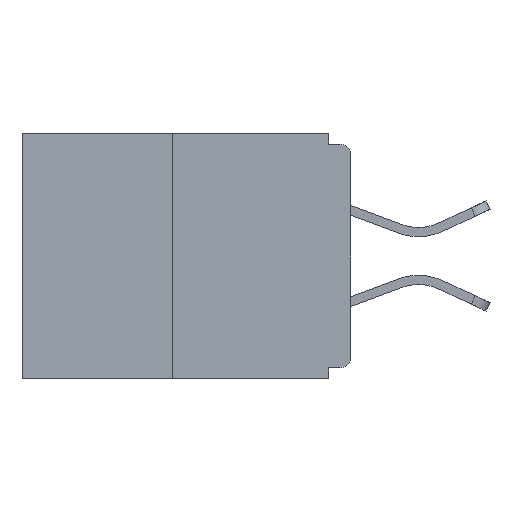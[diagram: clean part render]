
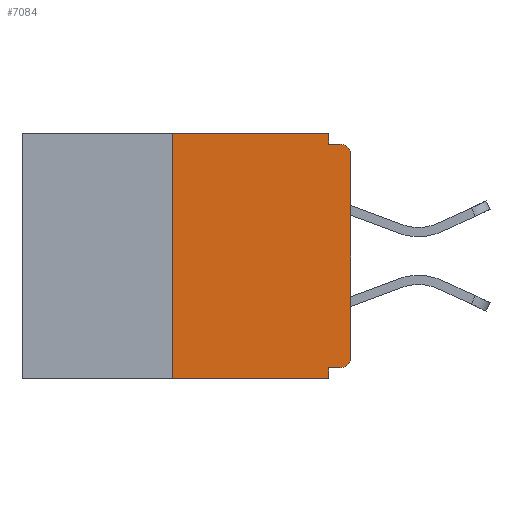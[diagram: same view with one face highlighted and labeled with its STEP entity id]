
A CAD part, left-side view. The second image highlights one B-rep face of the part: STEP entity #7084.
In plain terms, the highlighted planar face has unit normal (-1, 0, 0).
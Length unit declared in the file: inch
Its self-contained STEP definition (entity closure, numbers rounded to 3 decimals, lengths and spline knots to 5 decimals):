
#202 = DIRECTION ( 'NONE',  ( -1., 0., 0. ) ) ;
#292 = ORIENTED_EDGE ( 'NONE', *, *, #16657, .F. ) ;
#450 = EDGE_CURVE ( 'NONE', #7849, #12777, #5446, .T. ) ;
#792 = VECTOR ( 'NONE', #19011, 39.37008 ) ;
#882 = CARTESIAN_POINT ( 'NONE',  ( 0., 0.25, -0.343 ) ) ;
#975 = LINE ( 'NONE', #17782, #13413 ) ;
#1173 = VERTEX_POINT ( 'NONE', #20129 ) ;
#2070 = CARTESIAN_POINT ( 'NONE',  ( 0., 0.25, 0. ) ) ;
#2270 = ORIENTED_EDGE ( 'NONE', *, *, #19446, .T. ) ;
#2441 = LINE ( 'NONE', #14043, #18023 ) ;
#2995 = LINE ( 'NONE', #18815, #792 ) ;
#3107 = CARTESIAN_POINT ( 'NONE',  ( 0., 0.031, -0.015 ) ) ;
#3243 = DIRECTION ( 'NONE',  ( 0., 0., -1. ) ) ;
#3460 = ORIENTED_EDGE ( 'NONE', *, *, #10052, .F. ) ;
#3511 = LINE ( 'NONE', #4772, #19583 ) ;
#3733 = CARTESIAN_POINT ( 'NONE',  ( 0., 0.46, 0. ) ) ;
#3888 = DIRECTION ( 'NONE',  ( 0., -1., 0. ) ) ;
#3919 = VERTEX_POINT ( 'NONE', #2070 ) ;
#4026 = CARTESIAN_POINT ( 'NONE',  ( 0., 0.031, -0.328 ) ) ;
#4136 = CARTESIAN_POINT ( 'NONE',  ( 0., 0.031, -0.343 ) ) ;
#4229 = DIRECTION ( 'NONE',  ( 0., 0., -1. ) ) ;
#4297 = ORIENTED_EDGE ( 'NONE', *, *, #8947, .F. ) ;
#4772 = CARTESIAN_POINT ( 'NONE',  ( 0., 0.25, 0. ) ) ;
#4826 = CARTESIAN_POINT ( 'NONE',  ( 0., 0.015, -0.03 ) ) ;
#5094 = CARTESIAN_POINT ( 'NONE',  ( 0., 0.031, 0. ) ) ;
#5446 = LINE ( 'NONE', #12890, #10282 ) ;
#5510 = DIRECTION ( 'NONE',  ( 0., -1., 0. ) ) ;
#5558 = VERTEX_POINT ( 'NONE', #5094 ) ;
#5846 = DIRECTION ( 'NONE',  ( 0., 0., 1. ) ) ;
#5995 = LINE ( 'NONE', #3733, #7637 ) ;
#7084 = ADVANCED_FACE ( 'NONE', ( #8911 ), #7354, .F. ) ;
#7354 = PLANE ( 'NONE',  #11264 ) ;
#7637 = VECTOR ( 'NONE', #5510, 39.37008 ) ;
#7753 = ORIENTED_EDGE ( 'NONE', *, *, #10640, .T. ) ;
#7849 = VERTEX_POINT ( 'NONE', #4026 ) ;
#8017 = DIRECTION ( 'NONE',  ( 0., 0., -1. ) ) ;
#8213 = CIRCLE ( 'NONE', #14127, 0.015 ) ;
#8911 = FACE_OUTER_BOUND ( 'NONE', #9313, .T. ) ;
#8920 = DIRECTION ( 'NONE',  ( 1., 0., 0. ) ) ;
#8947 = EDGE_CURVE ( 'NONE', #5558, #17525, #2995, .T. ) ;
#9313 = EDGE_LOOP ( 'NONE', ( #19508, #11235, #11438, #16617, #3460, #2270, #7753, #10214, #292, #4297 ) ) ;
#9475 = DIRECTION ( 'NONE',  ( -1., 0., 0. ) ) ;
#9609 = DIRECTION ( 'NONE',  ( 0., -1., 0. ) ) ;
#9610 = CARTESIAN_POINT ( 'NONE',  ( 0., 0.015, -0.313 ) ) ;
#10051 = AXIS2_PLACEMENT_3D ( 'NONE', #4826, #202, #8017 ) ;
#10052 = EDGE_CURVE ( 'NONE', #14212, #7849, #2441, .T. ) ;
#10214 = ORIENTED_EDGE ( 'NONE', *, *, #18427, .T. ) ;
#10282 = VECTOR ( 'NONE', #17563, 39.37008 ) ;
#10444 = CARTESIAN_POINT ( 'NONE',  ( 0., 0., 0. ) ) ;
#10468 = EDGE_CURVE ( 'NONE', #3919, #5558, #5995, .T. ) ;
#10640 = EDGE_CURVE ( 'NONE', #1173, #11340, #11341, .T. ) ;
#11235 = ORIENTED_EDGE ( 'NONE', *, *, #15043, .F. ) ;
#11264 = AXIS2_PLACEMENT_3D ( 'NONE', #11999, #8920, #4229 ) ;
#11340 = VERTEX_POINT ( 'NONE', #19277 ) ;
#11341 = LINE ( 'NONE', #10444, #20094 ) ;
#11438 = ORIENTED_EDGE ( 'NONE', *, *, #13211, .T. ) ;
#11776 = CARTESIAN_POINT ( 'NONE',  ( 0., 0.015, -0.328 ) ) ;
#11999 = CARTESIAN_POINT ( 'NONE',  ( 0., 0.46, 0. ) ) ;
#12569 = VERTEX_POINT ( 'NONE', #882 ) ;
#12777 = VERTEX_POINT ( 'NONE', #4136 ) ;
#12890 = CARTESIAN_POINT ( 'NONE',  ( 0., 0.031, -0.343 ) ) ;
#13211 = EDGE_CURVE ( 'NONE', #12569, #12777, #18056, .T. ) ;
#13408 = VERTEX_POINT ( 'NONE', #16350 ) ;
#13413 = VECTOR ( 'NONE', #3888, 39.37008 ) ;
#13891 = CIRCLE ( 'NONE', #10051, 0.015 ) ;
#13909 = DIRECTION ( 'NONE',  ( 0., 1., 0. ) ) ;
#14043 = CARTESIAN_POINT ( 'NONE',  ( 0., 0., -0.328 ) ) ;
#14127 = AXIS2_PLACEMENT_3D ( 'NONE', #9610, #9475, #3243 ) ;
#14212 = VERTEX_POINT ( 'NONE', #11776 ) ;
#15043 = EDGE_CURVE ( 'NONE', #12569, #3919, #3511, .T. ) ;
#15950 = CARTESIAN_POINT ( 'NONE',  ( 0., 0.46, -0.343 ) ) ;
#16350 = CARTESIAN_POINT ( 'NONE',  ( 0., 0.015, -0.015 ) ) ;
#16617 = ORIENTED_EDGE ( 'NONE', *, *, #450, .F. ) ;
#16657 = EDGE_CURVE ( 'NONE', #17525, #13408, #975, .T. ) ;
#17525 = VERTEX_POINT ( 'NONE', #3107 ) ;
#17552 = VECTOR ( 'NONE', #9609, 39.37008 ) ;
#17563 = DIRECTION ( 'NONE',  ( 0., 0., -1. ) ) ;
#17782 = CARTESIAN_POINT ( 'NONE',  ( 0., 0., -0.015 ) ) ;
#18023 = VECTOR ( 'NONE', #13909, 39.37008 ) ;
#18056 = LINE ( 'NONE', #15950, #17552 ) ;
#18427 = EDGE_CURVE ( 'NONE', #11340, #13408, #13891, .T. ) ;
#18626 = DIRECTION ( 'NONE',  ( 0., 0., 1. ) ) ;
#18815 = CARTESIAN_POINT ( 'NONE',  ( 0., 0.031, 0. ) ) ;
#19011 = DIRECTION ( 'NONE',  ( 0., 0., -1. ) ) ;
#19277 = CARTESIAN_POINT ( 'NONE',  ( 0., 0., -0.03 ) ) ;
#19446 = EDGE_CURVE ( 'NONE', #14212, #1173, #8213, .T. ) ;
#19508 = ORIENTED_EDGE ( 'NONE', *, *, #10468, .F. ) ;
#19583 = VECTOR ( 'NONE', #18626, 39.37008 ) ;
#20094 = VECTOR ( 'NONE', #5846, 39.37008 ) ;
#20129 = CARTESIAN_POINT ( 'NONE',  ( 0., 0., -0.313 ) ) ;
